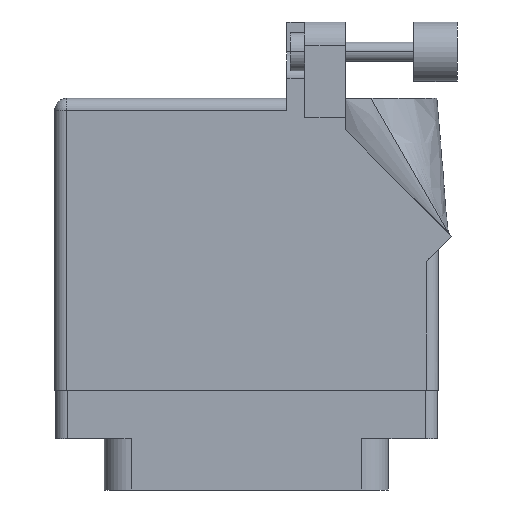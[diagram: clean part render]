
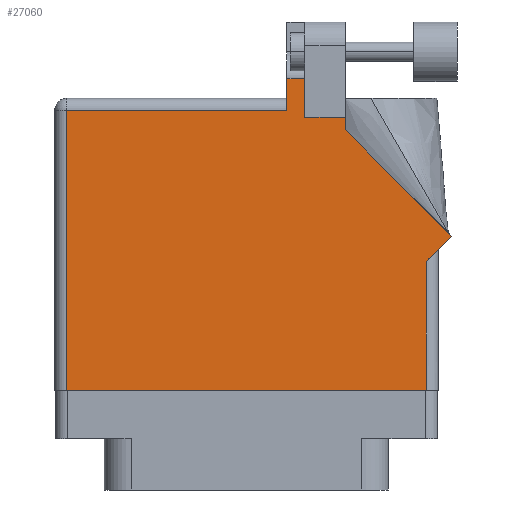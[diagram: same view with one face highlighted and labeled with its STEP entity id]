
A CAD part, front view. The second image highlights one B-rep face of the part: STEP entity #27060.
In plain terms, the highlighted face is planar.
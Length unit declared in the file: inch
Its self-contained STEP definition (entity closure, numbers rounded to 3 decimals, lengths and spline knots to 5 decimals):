
#335 = VERTEX_POINT ( 'NONE', #13739 ) ;
#895 = CARTESIAN_POINT ( 'NONE',  ( -1.005, -0.1, 0.455 ) ) ;
#1593 = EDGE_CURVE ( 'NONE', #21621, #24366, #23218, .T. ) ;
#2860 = EDGE_CURVE ( 'NONE', #23221, #27081, #12444, .T. ) ;
#2913 = VERTEX_POINT ( 'NONE', #9099 ) ;
#3101 = LINE ( 'NONE', #13488, #17596 ) ;
#3444 = VERTEX_POINT ( 'NONE', #26770 ) ;
#3855 = DIRECTION ( 'NONE',  ( 0., 1., 0. ) ) ;
#4685 = EDGE_CURVE ( 'NONE', #27081, #29927, #3101, .T. ) ;
#4876 = CARTESIAN_POINT ( 'NONE',  ( 0.519, 1.26442, 0.455 ) ) ;
#5146 = DIRECTION ( 'NONE',  ( -1., 0., 0. ) ) ;
#5293 = VECTOR ( 'NONE', #19628, 39.37008 ) ;
#5493 = VERTEX_POINT ( 'NONE', #15760 ) ;
#6387 = EDGE_CURVE ( 'NONE', #24366, #20540, #20939, .T. ) ;
#6919 = DIRECTION ( 'NONE',  ( -1., 0., 0. ) ) ;
#8002 = VECTOR ( 'NONE', #22631, 39.37008 ) ;
#8076 = CARTESIAN_POINT ( 'NONE',  ( 1.005, 0.637, 0.455 ) ) ;
#8458 = LINE ( 'NONE', #8792, #8002 ) ;
#8511 = CARTESIAN_POINT ( 'NONE',  ( -0.943, 1.368, 0.455 ) ) ;
#8792 = CARTESIAN_POINT ( 'NONE',  ( -0.943, -0.1, 0.455 ) ) ;
#9099 = CARTESIAN_POINT ( 'NONE',  ( 0.943, -0.1, 0.455 ) ) ;
#10749 = CARTESIAN_POINT ( 'NONE',  ( 0.943, 0.637, 0.455 ) ) ;
#11446 = CARTESIAN_POINT ( 'NONE',  ( 0.519, 1.33, 0.455 ) ) ;
#11667 = VECTOR ( 'NONE', #31279, 39.37008 ) ;
#12261 = CARTESIAN_POINT ( 'NONE',  ( 1.07571, 0.70771, 0.455 ) ) ;
#12444 = LINE ( 'NONE', #26314, #16810 ) ;
#12580 = CARTESIAN_POINT ( 'NONE',  ( 0.519, 1.26442, 0.455 ) ) ;
#12695 = LINE ( 'NONE', #33379, #34178 ) ;
#13217 = CARTESIAN_POINT ( 'NONE',  ( 0.943, 0.575, 0.455 ) ) ;
#13308 = DIRECTION ( 'NONE',  ( 0., 1., 0. ) ) ;
#13488 = CARTESIAN_POINT ( 'NONE',  ( -1.005, 1.368, 0.455 ) ) ;
#13739 = CARTESIAN_POINT ( 'NONE',  ( 0.306, 1.33, 0.455 ) ) ;
#15218 = CARTESIAN_POINT ( 'NONE',  ( 0.212, 1.5315, 0.455 ) ) ;
#15700 = EDGE_CURVE ( 'NONE', #335, #5493, #17068, .T. ) ;
#15719 = ORIENTED_EDGE ( 'NONE', *, *, #32741, .T. ) ;
#15760 = CARTESIAN_POINT ( 'NONE',  ( 0.306, 1.5315, 0.455 ) ) ;
#15834 = EDGE_CURVE ( 'NONE', #5493, #23221, #12695, .T. ) ;
#16043 = VECTOR ( 'NONE', #33263, 39.37008 ) ;
#16450 = LINE ( 'NONE', #895, #11667 ) ;
#16810 = VECTOR ( 'NONE', #34684, 39.37008 ) ;
#17068 = LINE ( 'NONE', #33963, #32335 ) ;
#17596 = VECTOR ( 'NONE', #5146, 39.37008 ) ;
#18831 = CARTESIAN_POINT ( 'NONE',  ( 1.07571, 0.70771, 0.455 ) ) ;
#19270 = VECTOR ( 'NONE', #24690, 39.37008 ) ;
#19628 = DIRECTION ( 'NONE',  ( -1., 0., 0. ) ) ;
#20540 = VERTEX_POINT ( 'NONE', #32187 ) ;
#20599 = PLANE ( 'NONE',  #20974 ) ;
#20730 = DIRECTION ( 'NONE',  ( 0., 0., -1. ) ) ;
#20939 = LINE ( 'NONE', #12580, #28834 ) ;
#20974 = AXIS2_PLACEMENT_3D ( 'NONE', #28924, #20730, #6919 ) ;
#21614 = VECTOR ( 'NONE', #13308, 39.37008 ) ;
#21621 = VERTEX_POINT ( 'NONE', #12261 ) ;
#21856 = DIRECTION ( 'NONE',  ( -1., 0., 0. ) ) ;
#22631 = DIRECTION ( 'NONE',  ( 0., -1., 0. ) ) ;
#22688 = ORIENTED_EDGE ( 'NONE', *, *, #15700, .T. ) ;
#23171 = DIRECTION ( 'NONE',  ( 0., 1., 0. ) ) ;
#23218 = LINE ( 'NONE', #18831, #19270 ) ;
#23221 = VERTEX_POINT ( 'NONE', #15218 ) ;
#23777 = ORIENTED_EDGE ( 'NONE', *, *, #30303, .T. ) ;
#23952 = ORIENTED_EDGE ( 'NONE', *, *, #32131, .T. ) ;
#24366 = VERTEX_POINT ( 'NONE', #4876 ) ;
#24690 = DIRECTION ( 'NONE',  ( -0.707, 0.707, 0. ) ) ;
#24734 = ORIENTED_EDGE ( 'NONE', *, *, #6387, .T. ) ;
#25743 = ORIENTED_EDGE ( 'NONE', *, *, #26858, .T. ) ;
#26008 = LINE ( 'NONE', #10749, #21614 ) ;
#26314 = CARTESIAN_POINT ( 'NONE',  ( 0.212, 1.43, 0.455 ) ) ;
#26770 = CARTESIAN_POINT ( 'NONE',  ( -0.943, -0.1, 0.455 ) ) ;
#26843 = CARTESIAN_POINT ( 'NONE',  ( 0.212, 1.368, 0.455 ) ) ;
#26858 = EDGE_CURVE ( 'NONE', #3444, #2913, #16450, .T. ) ;
#27060 = ADVANCED_FACE ( 'NONE', ( #35316 ), #20599, .F. ) ;
#27081 = VERTEX_POINT ( 'NONE', #26843 ) ;
#28688 = VERTEX_POINT ( 'NONE', #13217 ) ;
#28834 = VECTOR ( 'NONE', #3855, 39.37008 ) ;
#28924 = CARTESIAN_POINT ( 'NONE',  ( -1.005, 1.43, 0.455 ) ) ;
#29927 = VERTEX_POINT ( 'NONE', #8511 ) ;
#30203 = ORIENTED_EDGE ( 'NONE', *, *, #4685, .T. ) ;
#30303 = EDGE_CURVE ( 'NONE', #2913, #28688, #26008, .T. ) ;
#31279 = DIRECTION ( 'NONE',  ( 1., 0., 0. ) ) ;
#31446 = ORIENTED_EDGE ( 'NONE', *, *, #15834, .T. ) ;
#32131 = EDGE_CURVE ( 'NONE', #29927, #3444, #8458, .T. ) ;
#32187 = CARTESIAN_POINT ( 'NONE',  ( 0.519, 1.33, 0.455 ) ) ;
#32335 = VECTOR ( 'NONE', #23171, 39.37008 ) ;
#32741 = EDGE_CURVE ( 'NONE', #20540, #335, #34240, .T. ) ;
#33117 = LINE ( 'NONE', #8076, #16043 ) ;
#33137 = ORIENTED_EDGE ( 'NONE', *, *, #1593, .T. ) ;
#33263 = DIRECTION ( 'NONE',  ( 0.707, 0.707, 0. ) ) ;
#33379 = CARTESIAN_POINT ( 'NONE',  ( 0.63677, 1.5315, 0.455 ) ) ;
#33533 = EDGE_CURVE ( 'NONE', #28688, #21621, #33117, .T. ) ;
#33868 = ORIENTED_EDGE ( 'NONE', *, *, #33533, .T. ) ;
#33963 = CARTESIAN_POINT ( 'NONE',  ( 0.306, 1.33, 0.455 ) ) ;
#34178 = VECTOR ( 'NONE', #21856, 39.37008 ) ;
#34240 = LINE ( 'NONE', #11446, #5293 ) ;
#34383 = ORIENTED_EDGE ( 'NONE', *, *, #2860, .T. ) ;
#34684 = DIRECTION ( 'NONE',  ( 0., -1., 0. ) ) ;
#34738 = EDGE_LOOP ( 'NONE', ( #22688, #31446, #34383, #30203, #23952, #25743, #23777, #33868, #33137, #24734, #15719 ) ) ;
#35316 = FACE_OUTER_BOUND ( 'NONE', #34738, .T. ) ;
